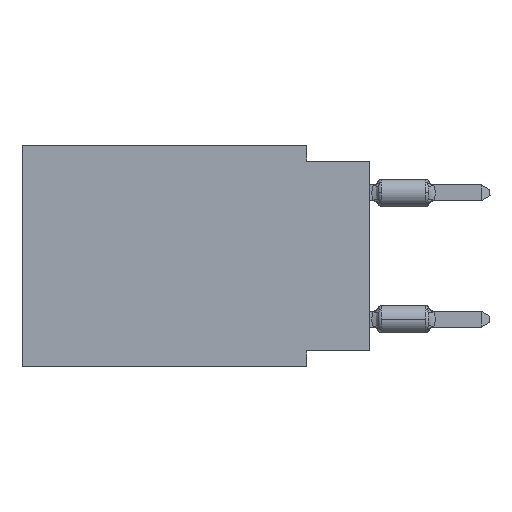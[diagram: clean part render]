
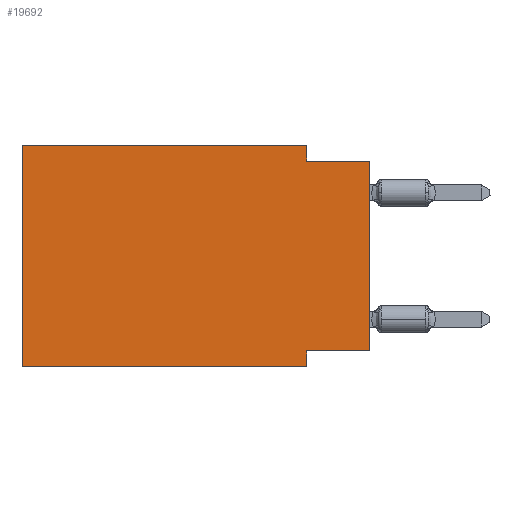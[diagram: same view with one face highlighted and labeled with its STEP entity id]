
A CAD part, left-side view. The second image highlights one B-rep face of the part: STEP entity #19692.
In plain terms, the highlighted planar face has unit normal (-1, 0, 0).
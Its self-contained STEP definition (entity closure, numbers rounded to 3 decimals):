
#81 = EDGE_LOOP ( 'NONE', ( #23222, #24220, #38001, #19240, #24253, #31976, #20603, #25476 ) ) ;
#1742 = DIRECTION ( 'NONE',  ( 0., 0., -1. ) ) ;
#2617 = CARTESIAN_POINT ( 'NONE',  ( 0., 0., -8.255 ) ) ;
#2980 = VERTEX_POINT ( 'NONE', #2617 ) ;
#3380 = CARTESIAN_POINT ( 'NONE',  ( 0., 13.97, -8.89 ) ) ;
#3962 = LINE ( 'NONE', #20645, #44976 ) ;
#5929 = VERTEX_POINT ( 'NONE', #3380 ) ;
#8398 = DIRECTION ( 'NONE',  ( 0., 0., 1. ) ) ;
#8439 = LINE ( 'NONE', #8968, #40617 ) ;
#8507 = CARTESIAN_POINT ( 'NONE',  ( 0., 13.97, -8.89 ) ) ;
#8556 = EDGE_CURVE ( 'NONE', #42405, #38095, #8664, .T. ) ;
#8664 = LINE ( 'NONE', #49886, #32819 ) ;
#8701 = DIRECTION ( 'NONE',  ( 0., -1., 0. ) ) ;
#8968 = CARTESIAN_POINT ( 'NONE',  ( 0., 0., -0.635 ) ) ;
#9182 = LINE ( 'NONE', #34022, #23534 ) ;
#10788 = VERTEX_POINT ( 'NONE', #24172 ) ;
#11773 = LINE ( 'NONE', #33589, #34923 ) ;
#12481 = CARTESIAN_POINT ( 'NONE',  ( 0., 0., 0. ) ) ;
#12486 = DIRECTION ( 'NONE',  ( 0., -1., 0. ) ) ;
#13373 = EDGE_CURVE ( 'NONE', #2980, #15178, #9182, .T. ) ;
#14179 = VERTEX_POINT ( 'NONE', #43750 ) ;
#15178 = VERTEX_POINT ( 'NONE', #35444 ) ;
#16196 = DIRECTION ( 'NONE',  ( 1., 0., 0. ) ) ;
#16534 = DIRECTION ( 'NONE',  ( 0., 0., 1. ) ) ;
#18076 = EDGE_CURVE ( 'NONE', #5929, #14179, #45906, .T. ) ;
#18363 = EDGE_CURVE ( 'NONE', #10788, #47635, #8439, .T. ) ;
#19240 = ORIENTED_EDGE ( 'NONE', *, *, #8556, .F. ) ;
#19692 = ADVANCED_FACE ( 'NONE', ( #24381 ), #41023, .F. ) ;
#20603 = ORIENTED_EDGE ( 'NONE', *, *, #20901, .F. ) ;
#20645 = CARTESIAN_POINT ( 'NONE',  ( 0., 13.97, 0. ) ) ;
#20901 = EDGE_CURVE ( 'NONE', #15178, #14179, #35619, .T. ) ;
#21029 = DIRECTION ( 'NONE',  ( 0., 0., -1. ) ) ;
#23222 = ORIENTED_EDGE ( 'NONE', *, *, #37288, .T. ) ;
#23534 = VECTOR ( 'NONE', #33025, 1000. ) ;
#24172 = CARTESIAN_POINT ( 'NONE',  ( 0., 2.54, -0.635 ) ) ;
#24220 = ORIENTED_EDGE ( 'NONE', *, *, #18363, .F. ) ;
#24253 = ORIENTED_EDGE ( 'NONE', *, *, #37667, .F. ) ;
#24381 = FACE_OUTER_BOUND ( 'NONE', #81, .T. ) ;
#25476 = ORIENTED_EDGE ( 'NONE', *, *, #13373, .F. ) ;
#28699 = CARTESIAN_POINT ( 'NONE',  ( 0., 2.54, 0. ) ) ;
#30993 = VECTOR ( 'NONE', #41801, 1000. ) ;
#31199 = EDGE_CURVE ( 'NONE', #38095, #10788, #11773, .T. ) ;
#31976 = ORIENTED_EDGE ( 'NONE', *, *, #18076, .T. ) ;
#32819 = VECTOR ( 'NONE', #12486, 1000. ) ;
#32850 = DIRECTION ( 'NONE',  ( 0., 0., -1. ) ) ;
#33025 = DIRECTION ( 'NONE',  ( 0., 1., 0. ) ) ;
#33589 = CARTESIAN_POINT ( 'NONE',  ( 0., 2.54, 0. ) ) ;
#34022 = CARTESIAN_POINT ( 'NONE',  ( 0., 0., -8.255 ) ) ;
#34649 = VECTOR ( 'NONE', #1742, 1000. ) ;
#34923 = VECTOR ( 'NONE', #21029, 1000. ) ;
#35444 = CARTESIAN_POINT ( 'NONE',  ( 0., 2.54, -8.255 ) ) ;
#35619 = LINE ( 'NONE', #43263, #34649 ) ;
#36929 = CARTESIAN_POINT ( 'NONE',  ( 0., 13.97, 0. ) ) ;
#37288 = EDGE_CURVE ( 'NONE', #2980, #47635, #45012, .T. ) ;
#37667 = EDGE_CURVE ( 'NONE', #5929, #42405, #3962, .T. ) ;
#38001 = ORIENTED_EDGE ( 'NONE', *, *, #31199, .F. ) ;
#38095 = VERTEX_POINT ( 'NONE', #28699 ) ;
#40617 = VECTOR ( 'NONE', #8701, 1000. ) ;
#41023 = PLANE ( 'NONE',  #46756 ) ;
#41801 = DIRECTION ( 'NONE',  ( 0., -1., 0. ) ) ;
#42405 = VERTEX_POINT ( 'NONE', #49450 ) ;
#43263 = CARTESIAN_POINT ( 'NONE',  ( 0., 2.54, -8.89 ) ) ;
#43750 = CARTESIAN_POINT ( 'NONE',  ( 0., 2.54, -8.89 ) ) ;
#44389 = CARTESIAN_POINT ( 'NONE',  ( 0., 0., -0.635 ) ) ;
#44976 = VECTOR ( 'NONE', #16534, 1000. ) ;
#45012 = LINE ( 'NONE', #12481, #46666 ) ;
#45906 = LINE ( 'NONE', #8507, #30993 ) ;
#46666 = VECTOR ( 'NONE', #8398, 1000. ) ;
#46756 = AXIS2_PLACEMENT_3D ( 'NONE', #36929, #16196, #32850 ) ;
#47635 = VERTEX_POINT ( 'NONE', #44389 ) ;
#49450 = CARTESIAN_POINT ( 'NONE',  ( 0., 13.97, 0. ) ) ;
#49886 = CARTESIAN_POINT ( 'NONE',  ( 0., 13.97, 0. ) ) ;
